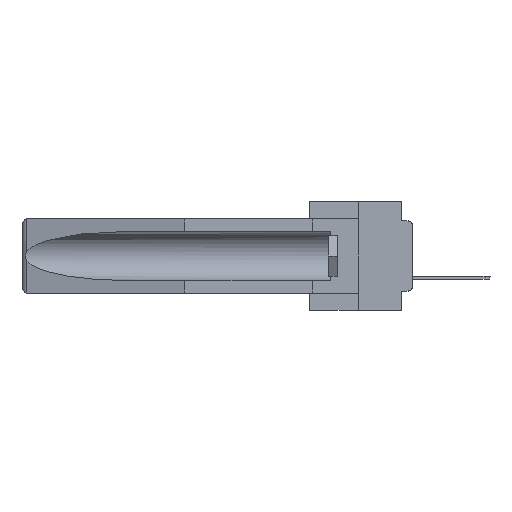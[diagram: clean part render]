
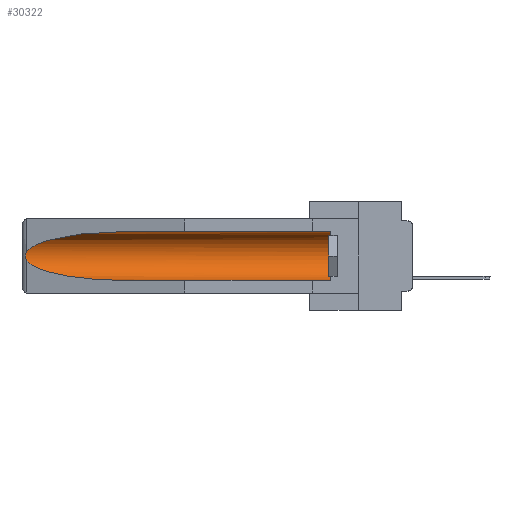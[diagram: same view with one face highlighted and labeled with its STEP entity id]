
A CAD part, left-side view. The second image highlights one B-rep face of the part: STEP entity #30322.
In plain terms, the highlighted cylindrical face has radius 2.857 mm (diameter 5.715 mm), a partial arc.
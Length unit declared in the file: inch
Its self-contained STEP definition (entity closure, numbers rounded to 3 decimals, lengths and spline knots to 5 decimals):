
#201 = ORIENTED_EDGE ( 'NONE', *, *, #29226, .T. ) ;
#3847 = EDGE_CURVE ( 'NONE', #30802, #30679, #33883, .T. ) ;
#3890 = CARTESIAN_POINT ( 'NONE',  ( 0.26537, 1.52718, -0.19328 ) ) ;
#4084 = CARTESIAN_POINT ( 'NONE',  ( 0.26537, 1.52718, -0.19328 ) ) ;
#5752 = CARTESIAN_POINT ( 'NONE',  ( 0.155, 1.07973, -0.059 ) ) ;
#6194 = CARTESIAN_POINT ( 'NONE',  ( 0.26537, 1.52718, -0.14972 ) ) ;
#6523 = CARTESIAN_POINT ( 'NONE',  ( 0.26654, 1.53092, -0.15636 ) ) ;
#6700 = VECTOR ( 'NONE', #23160, 39.37008 ) ;
#7457 = DIRECTION ( 'NONE',  ( 0., 1., 0. ) ) ;
#7823 = AXIS2_PLACEMENT_3D ( 'NONE', #8772, #19824, #28076 ) ;
#7912 = CARTESIAN_POINT ( 'NONE',  ( 0.26537, 1.52718, -0.14972 ) ) ;
#8380 = ORIENTED_EDGE ( 'NONE', *, *, #3847, .T. ) ;
#8772 = CARTESIAN_POINT ( 'NONE',  ( 0.155, 0.126, -0.1715 ) ) ;
#9345 = CARTESIAN_POINT ( 'NONE',  ( 0.2673, 1.53269, -0.17917 ) ) ;
#9355 = CARTESIAN_POINT ( 'NONE',  ( 0.25451, 1.48313, -0.24835 ) ) ;
#9484 = VERTEX_POINT ( 'NONE', #31472 ) ;
#10086 =( BOUNDED_CURVE ( )  B_SPLINE_CURVE ( 3, ( #10737, #21432, #29841, #7912 ),
 .UNSPECIFIED., .F., .T. ) 
 B_SPLINE_CURVE_WITH_KNOTS ( ( 4, 4 ),
 ( 4.71239, 6.08839 ),
 .UNSPECIFIED. ) 
 CURVE ( )  GEOMETRIC_REPRESENTATION_ITEM ( )  RATIONAL_B_SPLINE_CURVE ( ( 1., 0.848, 0.848, 1. ) ) 
 REPRESENTATION_ITEM ( '' )  );
#10276 = DIRECTION ( 'NONE',  ( 0., 1., 0. ) ) ;
#10737 = CARTESIAN_POINT ( 'NONE',  ( 0.155, 1.07973, -0.059 ) ) ;
#11637 = CARTESIAN_POINT ( 'NONE',  ( 0.26597, 1.52961, -0.15275 ) ) ;
#12409 = DIRECTION ( 'NONE',  ( 0., 0., 1. ) ) ;
#12732 = CARTESIAN_POINT ( 'NONE',  ( 0.155, -0.30754, -0.284 ) ) ;
#14275 = ORIENTED_EDGE ( 'NONE', *, *, #32135, .T. ) ;
#14617 = CARTESIAN_POINT ( 'NONE',  ( 0.26537, 1.52718, -0.14972 ) ) ;
#15368 = CYLINDRICAL_SURFACE ( 'NONE', #16280, 0.1125 ) ;
#15680 = CIRCLE ( 'NONE', #7823, 0.1125 ) ;
#16197 = CARTESIAN_POINT ( 'NONE',  ( 0.26537, 1.52718, -0.19328 ) ) ;
#16280 = AXIS2_PLACEMENT_3D ( 'NONE', #28505, #7457, #12409 ) ;
#16732 = CARTESIAN_POINT ( 'NONE',  ( 0.2673, 1.5327, -0.16383 ) ) ;
#19713 = CARTESIAN_POINT ( 'NONE',  ( 0.26655, 1.53094, -0.18657 ) ) ;
#19824 = DIRECTION ( 'NONE',  ( 0., -1., 0. ) ) ;
#19848 = ORIENTED_EDGE ( 'NONE', *, *, #31842, .F. ) ;
#20080 = FACE_OUTER_BOUND ( 'NONE', #20727, .T. ) ;
#20126 = VERTEX_POINT ( 'NONE', #5752 ) ;
#20552 = ORIENTED_EDGE ( 'NONE', *, *, #23223, .T. ) ;
#20727 = EDGE_LOOP ( 'NONE', ( #201, #14275, #8380, #19848, #27939, #20552 ) ) ;
#21432 = CARTESIAN_POINT ( 'NONE',  ( 0.21114, 1.30732, -0.059 ) ) ;
#22623 = LINE ( 'NONE', #33182, #6700 ) ;
#23055 = CARTESIAN_POINT ( 'NONE',  ( 0.21114, 1.30732, -0.284 ) ) ;
#23160 = DIRECTION ( 'NONE',  ( 0., 1., 0. ) ) ;
#23222 = CARTESIAN_POINT ( 'NONE',  ( 0.155, 0.126, -0.284 ) ) ;
#23223 = EDGE_CURVE ( 'NONE', #9484, #20126, #22623, .T. ) ;
#23388 = CARTESIAN_POINT ( 'NONE',  ( 0.155, 1.07973, -0.284 ) ) ;
#24814 = CARTESIAN_POINT ( 'NONE',  ( 0.26597, 1.5296, -0.19026 ) ) ;
#24970 = CARTESIAN_POINT ( 'NONE',  ( 0.2675, 1.53308, -0.16763 ) ) ;
#26065 = VECTOR ( 'NONE', #10276, 39.37008 ) ;
#26557 = CARTESIAN_POINT ( 'NONE',  ( 0.155, 1.07973, -0.284 ) ) ;
#27939 = ORIENTED_EDGE ( 'NONE', *, *, #28003, .T. ) ;
#28003 = EDGE_CURVE ( 'NONE', #33578, #9484, #15680, .T. ) ;
#28076 = DIRECTION ( 'NONE',  ( 0., 0., 1. ) ) ;
#28505 = CARTESIAN_POINT ( 'NONE',  ( 0.155, -0.30754, -0.1715 ) ) ;
#29226 = EDGE_CURVE ( 'NONE', #20126, #30942, #10086, .T. ) ;
#29841 = CARTESIAN_POINT ( 'NONE',  ( 0.25451, 1.48313, -0.09465 ) ) ;
#30322 = ADVANCED_FACE ( 'NONE', ( #20080 ), #15368, .F. ) ;
#30326 = B_SPLINE_CURVE_WITH_KNOTS ( 'NONE', 3,
 ( #6194, #11637, #6523, #16732, #24970, #33389, #9345, #19713, #24814, #3890 ),
 .UNSPECIFIED., .F., .F.,
 ( 4, 2, 2, 2, 4 ),
 ( 0., 0.00029, 0.00058, 0.00087, 0.00117 ),
 .UNSPECIFIED. ) ;
#30679 = VERTEX_POINT ( 'NONE', #26557 ) ;
#30802 = VERTEX_POINT ( 'NONE', #16197 ) ;
#30942 = VERTEX_POINT ( 'NONE', #14617 ) ;
#31472 = CARTESIAN_POINT ( 'NONE',  ( 0.155, 0.126, -0.059 ) ) ;
#31673 = LINE ( 'NONE', #12732, #26065 ) ;
#31842 = EDGE_CURVE ( 'NONE', #33578, #30679, #31673, .T. ) ;
#32135 = EDGE_CURVE ( 'NONE', #30942, #30802, #30326, .T. ) ;
#33182 = CARTESIAN_POINT ( 'NONE',  ( 0.155, -0.30754, -0.059 ) ) ;
#33389 = CARTESIAN_POINT ( 'NONE',  ( 0.2675, 1.53308, -0.17534 ) ) ;
#33578 = VERTEX_POINT ( 'NONE', #23222 ) ;
#33883 =( BOUNDED_CURVE ( )  B_SPLINE_CURVE ( 3, ( #4084, #9355, #23055, #23388 ),
 .UNSPECIFIED., .F., .T. ) 
 B_SPLINE_CURVE_WITH_KNOTS ( ( 4, 4 ),
 ( 0.1948, 1.5708 ),
 .UNSPECIFIED. ) 
 CURVE ( )  GEOMETRIC_REPRESENTATION_ITEM ( )  RATIONAL_B_SPLINE_CURVE ( ( 1., 0.848, 0.848, 1. ) ) 
 REPRESENTATION_ITEM ( '' )  );
